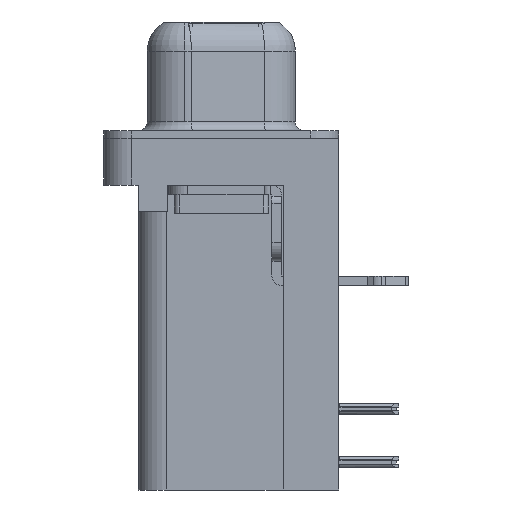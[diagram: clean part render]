
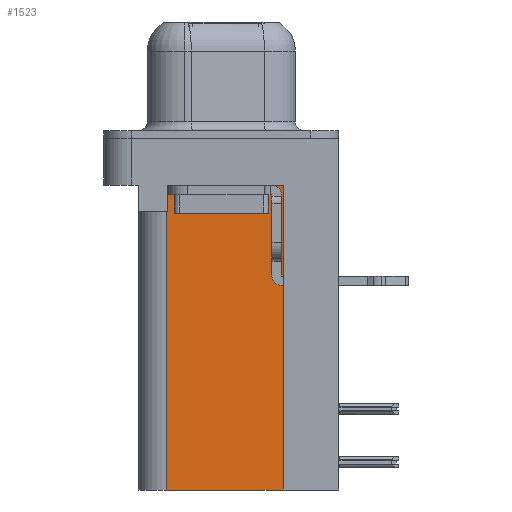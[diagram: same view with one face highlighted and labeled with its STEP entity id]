
A CAD part, left-side view. The second image highlights one B-rep face of the part: STEP entity #1523.
In plain terms, the highlighted planar face has unit normal (-1, 0, 0).
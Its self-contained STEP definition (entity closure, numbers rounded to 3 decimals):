
#1523 = ADVANCED_FACE ( 'NONE', ( #33429 ), #35131, .F. ) ;
#2873 = LINE ( 'NONE', #33896, #2904 ) ;
#2904 = VECTOR ( 'NONE', #17035, 1000. ) ;
#2908 = CARTESIAN_POINT ( 'NONE',  ( 3.79, -3.295, -18.76 ) ) ;
#4649 = ORIENTED_EDGE ( 'NONE', *, *, #24497, .F. ) ;
#5163 = CARTESIAN_POINT ( 'NONE',  ( 3.79, -3.295, -2.5 ) ) ;
#5465 = VERTEX_POINT ( 'NONE', #2908 ) ;
#5479 = ORIENTED_EDGE ( 'NONE', *, *, #6953, .T. ) ;
#5873 = DIRECTION ( 'NONE',  ( 0., 0., 1. ) ) ;
#6953 = EDGE_CURVE ( 'NONE', #21199, #10602, #14385, .T. ) ;
#7222 = DIRECTION ( 'NONE',  ( 0., 1., 0. ) ) ;
#8077 = CARTESIAN_POINT ( 'NONE',  ( 3.79, 2.895, -3.9 ) ) ;
#8329 = CARTESIAN_POINT ( 'NONE',  ( 3.79, 2.895, -3.9 ) ) ;
#8627 = LINE ( 'NONE', #24050, #24247 ) ;
#9610 = EDGE_CURVE ( 'NONE', #20814, #21199, #22465, .T. ) ;
#10602 = VERTEX_POINT ( 'NONE', #20067 ) ;
#11042 = LINE ( 'NONE', #22059, #11281 ) ;
#11281 = VECTOR ( 'NONE', #27680, 1000. ) ;
#11449 = DIRECTION ( 'NONE',  ( 0., 0., -1. ) ) ;
#12127 = VECTOR ( 'NONE', #27822, 1000. ) ;
#14385 = LINE ( 'NONE', #24974, #12127 ) ;
#14663 = CARTESIAN_POINT ( 'NONE',  ( 3.79, 2.895, -2.5 ) ) ;
#17035 = DIRECTION ( 'NONE',  ( 0., 1., 0. ) ) ;
#19257 = VECTOR ( 'NONE', #5873, 1000. ) ;
#19777 = LINE ( 'NONE', #23562, #19257 ) ;
#20067 = CARTESIAN_POINT ( 'NONE',  ( 3.79, 2.925, -3.9 ) ) ;
#20166 = VERTEX_POINT ( 'NONE', #5163 ) ;
#20814 = VERTEX_POINT ( 'NONE', #14663 ) ;
#21199 = VERTEX_POINT ( 'NONE', #8077 ) ;
#21417 = DIRECTION ( 'NONE',  ( 1., 0., 0. ) ) ;
#21466 = CARTESIAN_POINT ( 'NONE',  ( 3.79, -3.295, -18.76 ) ) ;
#22059 = CARTESIAN_POINT ( 'NONE',  ( 3.79, -3.295, -18.76 ) ) ;
#22347 = VECTOR ( 'NONE', #11449, 1000. ) ;
#22465 = LINE ( 'NONE', #8329, #22347 ) ;
#23562 = CARTESIAN_POINT ( 'NONE',  ( 3.79, 2.925, -18.76 ) ) ;
#23630 = EDGE_CURVE ( 'NONE', #5465, #20166, #11042, .T. ) ;
#24050 = CARTESIAN_POINT ( 'NONE',  ( 3.79, -3.295, -2.5 ) ) ;
#24247 = VECTOR ( 'NONE', #29763, 1000. ) ;
#24272 = ORIENTED_EDGE ( 'NONE', *, *, #34467, .F. ) ;
#24497 = EDGE_CURVE ( 'NONE', #5465, #25937, #2873, .T. ) ;
#24974 = CARTESIAN_POINT ( 'NONE',  ( 3.79, 0., -3.9 ) ) ;
#25937 = VERTEX_POINT ( 'NONE', #35219 ) ;
#27680 = DIRECTION ( 'NONE',  ( 0., 0., 1. ) ) ;
#27822 = DIRECTION ( 'NONE',  ( 0., 1., 0. ) ) ;
#28446 = ORIENTED_EDGE ( 'NONE', *, *, #28987, .T. ) ;
#28987 = EDGE_CURVE ( 'NONE', #20166, #20814, #8627, .T. ) ;
#29411 = EDGE_LOOP ( 'NONE', ( #28446, #35624, #5479, #24272, #4649, #32909 ) ) ;
#29763 = DIRECTION ( 'NONE',  ( 0., 1., 0. ) ) ;
#32909 = ORIENTED_EDGE ( 'NONE', *, *, #23630, .T. ) ;
#33179 = AXIS2_PLACEMENT_3D ( 'NONE', #21466, #21417, #7222 ) ;
#33429 = FACE_OUTER_BOUND ( 'NONE', #29411, .T. ) ;
#33896 = CARTESIAN_POINT ( 'NONE',  ( 3.79, -3.295, -18.76 ) ) ;
#34467 = EDGE_CURVE ( 'NONE', #25937, #10602, #19777, .T. ) ;
#35131 = PLANE ( 'NONE',  #33179 ) ;
#35219 = CARTESIAN_POINT ( 'NONE',  ( 3.79, 2.925, -18.76 ) ) ;
#35624 = ORIENTED_EDGE ( 'NONE', *, *, #9610, .T. ) ;
